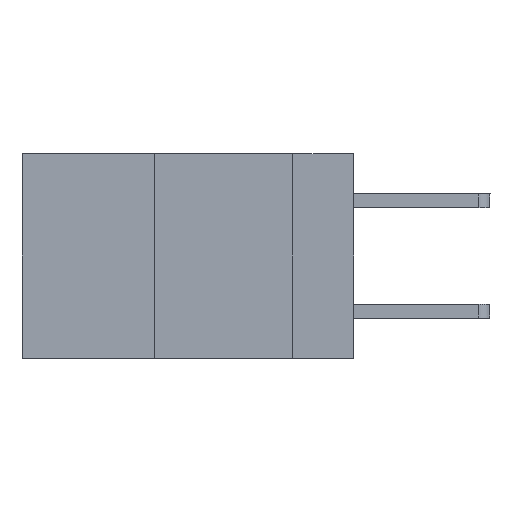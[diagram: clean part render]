
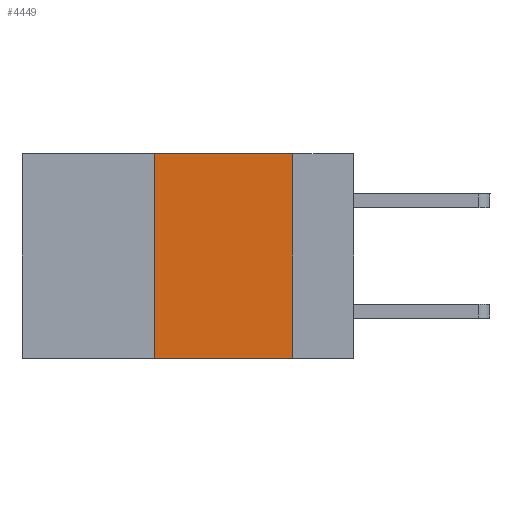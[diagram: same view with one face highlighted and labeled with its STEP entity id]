
A CAD part, left-side view. The second image highlights one B-rep face of the part: STEP entity #4449.
In plain terms, the highlighted planar face has unit normal (-1, 0, 0).
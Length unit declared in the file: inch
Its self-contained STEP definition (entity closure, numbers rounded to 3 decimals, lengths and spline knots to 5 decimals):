
#11 = DIRECTION ( 'NONE',  ( 0., 0., -1. ) ) ;
#42 = DIRECTION ( 'NONE',  ( 1., 0., 0. ) ) ;
#187 = LINE ( 'NONE', #5846, #9491 ) ;
#197 = PLANE ( 'NONE',  #4980 ) ;
#206 = VECTOR ( 'NONE', #7597, 39.37008 ) ;
#472 = CARTESIAN_POINT ( 'NONE',  ( 0., 0.36, -0.37 ) ) ;
#557 = EDGE_CURVE ( 'NONE', #6461, #9546, #2990, .T. ) ;
#598 = VECTOR ( 'NONE', #3812, 39.37008 ) ;
#2011 = EDGE_CURVE ( 'NONE', #9546, #4028, #9218, .T. ) ;
#2502 = EDGE_LOOP ( 'NONE', ( #3828, #3842, #3855, #3868 ) ) ;
#2802 = CARTESIAN_POINT ( 'NONE',  ( 0., 0.11, -0.37 ) ) ;
#2814 = LINE ( 'NONE', #5735, #598 ) ;
#2990 = LINE ( 'NONE', #8461, #206 ) ;
#3066 = DIRECTION ( 'NONE',  ( 0., 0., 1. ) ) ;
#3364 = VERTEX_POINT ( 'NONE', #472 ) ;
#3812 = DIRECTION ( 'NONE',  ( 0., -1., 0. ) ) ;
#3828 = ORIENTED_EDGE ( 'NONE', *, *, #2011, .F. ) ;
#3842 = ORIENTED_EDGE ( 'NONE', *, *, #557, .F. ) ;
#3855 = ORIENTED_EDGE ( 'NONE', *, *, #9626, .F. ) ;
#3868 = ORIENTED_EDGE ( 'NONE', *, *, #10361, .T. ) ;
#4028 = VERTEX_POINT ( 'NONE', #2802 ) ;
#4449 = ADVANCED_FACE ( 'NONE', ( #10081 ), #197, .F. ) ;
#4670 = CARTESIAN_POINT ( 'NONE',  ( 0., 0.6, 0. ) ) ;
#4735 = DIRECTION ( 'NONE',  ( 0., 0., -1. ) ) ;
#4760 = CARTESIAN_POINT ( 'NONE',  ( 0., 0.11, 0. ) ) ;
#4980 = AXIS2_PLACEMENT_3D ( 'NONE', #4670, #42, #11 ) ;
#5450 = CARTESIAN_POINT ( 'NONE',  ( 0., 0.36, 0. ) ) ;
#5470 = VECTOR ( 'NONE', #4735, 39.37008 ) ;
#5735 = CARTESIAN_POINT ( 'NONE',  ( 0., 0.6, -0.37 ) ) ;
#5846 = CARTESIAN_POINT ( 'NONE',  ( 0., 0.36, 0. ) ) ;
#6461 = VERTEX_POINT ( 'NONE', #5450 ) ;
#7597 = DIRECTION ( 'NONE',  ( 0., -1., 0. ) ) ;
#8461 = CARTESIAN_POINT ( 'NONE',  ( 0., 0.6, 0. ) ) ;
#9218 = LINE ( 'NONE', #4760, #5470 ) ;
#9491 = VECTOR ( 'NONE', #3066, 39.37008 ) ;
#9546 = VERTEX_POINT ( 'NONE', #10809 ) ;
#9626 = EDGE_CURVE ( 'NONE', #3364, #6461, #187, .T. ) ;
#10081 = FACE_OUTER_BOUND ( 'NONE', #2502, .T. ) ;
#10361 = EDGE_CURVE ( 'NONE', #3364, #4028, #2814, .T. ) ;
#10809 = CARTESIAN_POINT ( 'NONE',  ( 0., 0.11, 0. ) ) ;
